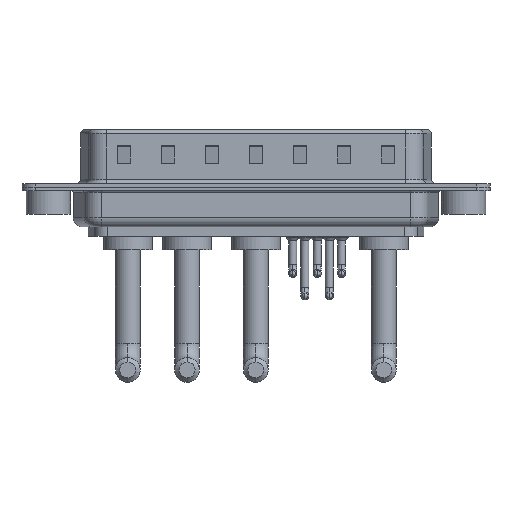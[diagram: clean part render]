
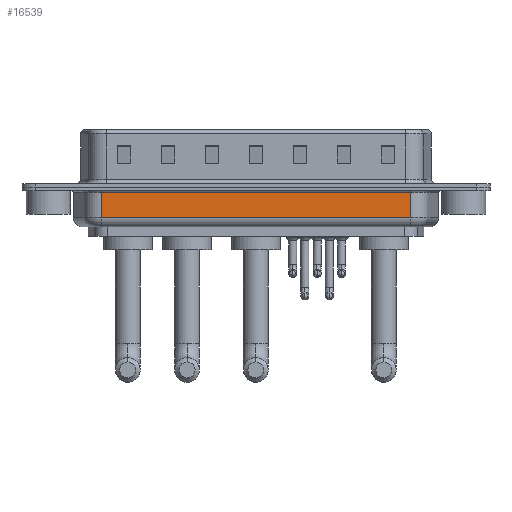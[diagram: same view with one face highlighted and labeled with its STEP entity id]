
A CAD part, front view. The second image highlights one B-rep face of the part: STEP entity #16539.
In plain terms, the highlighted planar face has unit normal (0, -1, 0).
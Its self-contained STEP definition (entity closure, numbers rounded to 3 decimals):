
#260 = CARTESIAN_POINT ( 'NONE',  ( 41.044, -5.35, -4.5 ) ) ;
#839 = EDGE_CURVE ( 'NONE', #20330, #5289, #15315, .T. ) ;
#1280 = CARTESIAN_POINT ( 'NONE',  ( 6.006, -5.35, -4.5 ) ) ;
#2250 = LINE ( 'NONE', #14462, #22292 ) ;
#3845 = EDGE_CURVE ( 'NONE', #14747, #7397, #20973, .T. ) ;
#4083 = DIRECTION ( 'NONE',  ( -1., 0., 0. ) ) ;
#4342 = CARTESIAN_POINT ( 'NONE',  ( 6.006, -5.35, -0.65 ) ) ;
#4705 = CARTESIAN_POINT ( 'NONE',  ( 6.006, -5.35, -4.5 ) ) ;
#5289 = VERTEX_POINT ( 'NONE', #4342 ) ;
#5718 = EDGE_CURVE ( 'NONE', #7397, #5289, #2250, .T. ) ;
#6199 = FACE_OUTER_BOUND ( 'NONE', #21659, .T. ) ;
#7397 = VERTEX_POINT ( 'NONE', #18975 ) ;
#7783 = PLANE ( 'NONE',  #20369 ) ;
#8228 = CARTESIAN_POINT ( 'NONE',  ( 41.044, -5.35, -3.5 ) ) ;
#8990 = VECTOR ( 'NONE', #20653, 1000. ) ;
#9209 = CARTESIAN_POINT ( 'NONE',  ( 6.006, -5.35, -3.5 ) ) ;
#9371 = DIRECTION ( 'NONE',  ( 1., 0., 0. ) ) ;
#10526 = VECTOR ( 'NONE', #15526, 1000. ) ;
#11153 = EDGE_CURVE ( 'NONE', #20330, #14747, #21333, .T. ) ;
#11414 = ORIENTED_EDGE ( 'NONE', *, *, #11153, .T. ) ;
#12125 = ORIENTED_EDGE ( 'NONE', *, *, #3845, .T. ) ;
#12177 = ORIENTED_EDGE ( 'NONE', *, *, #839, .F. ) ;
#14166 = ORIENTED_EDGE ( 'NONE', *, *, #5718, .T. ) ;
#14462 = CARTESIAN_POINT ( 'NONE',  ( 6.006, -5.35, -0.65 ) ) ;
#14747 = VERTEX_POINT ( 'NONE', #8228 ) ;
#15074 = DIRECTION ( 'NONE',  ( 0., 1., 0. ) ) ;
#15315 = LINE ( 'NONE', #4705, #8990 ) ;
#15526 = DIRECTION ( 'NONE',  ( 0., 0., 1. ) ) ;
#15886 = CARTESIAN_POINT ( 'NONE',  ( 6.006, -5.35, -3.5 ) ) ;
#16539 = ADVANCED_FACE ( 'NONE', ( #6199 ), #7783, .F. ) ;
#18480 = DIRECTION ( 'NONE',  ( 0., 0., 1. ) ) ;
#18975 = CARTESIAN_POINT ( 'NONE',  ( 41.044, -5.35, -0.65 ) ) ;
#19183 = VECTOR ( 'NONE', #9371, 1000. ) ;
#20330 = VERTEX_POINT ( 'NONE', #9209 ) ;
#20369 = AXIS2_PLACEMENT_3D ( 'NONE', #1280, #15074, #18480 ) ;
#20653 = DIRECTION ( 'NONE',  ( 0., 0., 1. ) ) ;
#20973 = LINE ( 'NONE', #260, #10526 ) ;
#21333 = LINE ( 'NONE', #15886, #19183 ) ;
#21659 = EDGE_LOOP ( 'NONE', ( #12177, #11414, #12125, #14166 ) ) ;
#22292 = VECTOR ( 'NONE', #4083, 1000. ) ;
